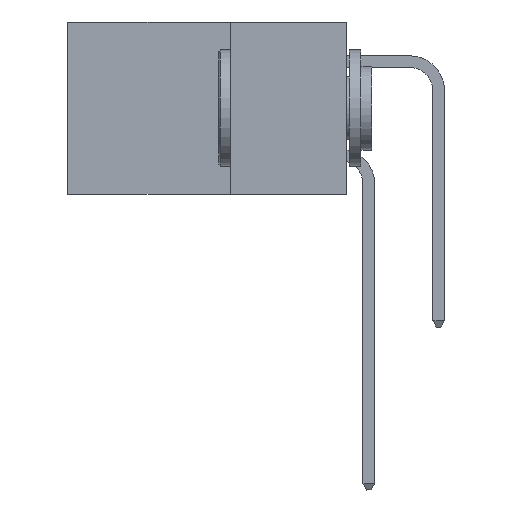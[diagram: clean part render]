
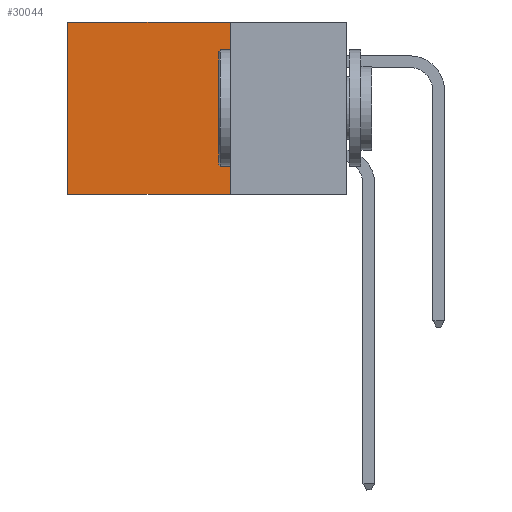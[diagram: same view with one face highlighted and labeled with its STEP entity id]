
A CAD part, left-side view. The second image highlights one B-rep face of the part: STEP entity #30044.
In plain terms, the highlighted planar face has unit normal (-1, 0, 0).
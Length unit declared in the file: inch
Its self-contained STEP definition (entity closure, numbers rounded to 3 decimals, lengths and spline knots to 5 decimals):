
#577 = DIRECTION ( 'NONE',  ( 0., 0., -1. ) ) ;
#609 = ORIENTED_EDGE ( 'NONE', *, *, #22271, .T. ) ;
#923 = EDGE_CURVE ( 'NONE', #34113, #4904, #39827, .T. ) ;
#1180 = CARTESIAN_POINT ( 'NONE',  ( 0.2875, 0.25, 0. ) ) ;
#2294 = EDGE_CURVE ( 'NONE', #7679, #27441, #3477, .T. ) ;
#2825 = DIRECTION ( 'NONE',  ( 0., 1., 0. ) ) ;
#3477 = LINE ( 'NONE', #1180, #27460 ) ;
#3893 = DIRECTION ( 'NONE',  ( 0., 0., -1. ) ) ;
#4904 = VERTEX_POINT ( 'NONE', #22905 ) ;
#5271 = ORIENTED_EDGE ( 'NONE', *, *, #923, .T. ) ;
#5279 = LINE ( 'NONE', #35071, #6248 ) ;
#5826 = ORIENTED_EDGE ( 'NONE', *, *, #2294, .F. ) ;
#6248 = VECTOR ( 'NONE', #22998, 39.37008 ) ;
#6843 = LINE ( 'NONE', #18266, #38653 ) ;
#7679 = VERTEX_POINT ( 'NONE', #31674 ) ;
#9389 = AXIS2_PLACEMENT_3D ( 'NONE', #38034, #31593, #577 ) ;
#11018 = EDGE_LOOP ( 'NONE', ( #5271, #37579, #5826, #609 ) ) ;
#16153 = PLANE ( 'NONE',  #9389 ) ;
#18266 = CARTESIAN_POINT ( 'NONE',  ( 0.2875, 0.25, -0.37 ) ) ;
#22176 = VECTOR ( 'NONE', #24032, 39.37008 ) ;
#22271 = EDGE_CURVE ( 'NONE', #7679, #34113, #5279, .T. ) ;
#22905 = CARTESIAN_POINT ( 'NONE',  ( 0.2875, 0.6, -0.37 ) ) ;
#22998 = DIRECTION ( 'NONE',  ( 0., 1., 0. ) ) ;
#24032 = DIRECTION ( 'NONE',  ( 0., 0., -1. ) ) ;
#27441 = VERTEX_POINT ( 'NONE', #27849 ) ;
#27460 = VECTOR ( 'NONE', #3893, 39.37008 ) ;
#27849 = CARTESIAN_POINT ( 'NONE',  ( 0.2875, 0.25, -0.37 ) ) ;
#30044 = ADVANCED_FACE ( 'NONE', ( #30642 ), #16153, .F. ) ;
#30642 = FACE_OUTER_BOUND ( 'NONE', #11018, .T. ) ;
#31593 = DIRECTION ( 'NONE',  ( 1., 0., 0. ) ) ;
#31674 = CARTESIAN_POINT ( 'NONE',  ( 0.2875, 0.25, 0. ) ) ;
#33219 = CARTESIAN_POINT ( 'NONE',  ( 0.2875, 0.6, 0. ) ) ;
#34113 = VERTEX_POINT ( 'NONE', #33219 ) ;
#35071 = CARTESIAN_POINT ( 'NONE',  ( 0.2875, 0.25, 0. ) ) ;
#37579 = ORIENTED_EDGE ( 'NONE', *, *, #38136, .F. ) ;
#38034 = CARTESIAN_POINT ( 'NONE',  ( 0.2875, 0.25, 0. ) ) ;
#38136 = EDGE_CURVE ( 'NONE', #27441, #4904, #6843, .T. ) ;
#38653 = VECTOR ( 'NONE', #2825, 39.37008 ) ;
#39505 = CARTESIAN_POINT ( 'NONE',  ( 0.2875, 0.6, 0. ) ) ;
#39827 = LINE ( 'NONE', #39505, #22176 ) ;
